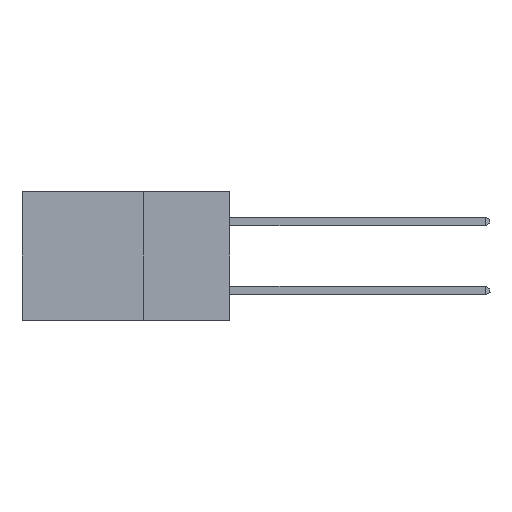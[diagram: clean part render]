
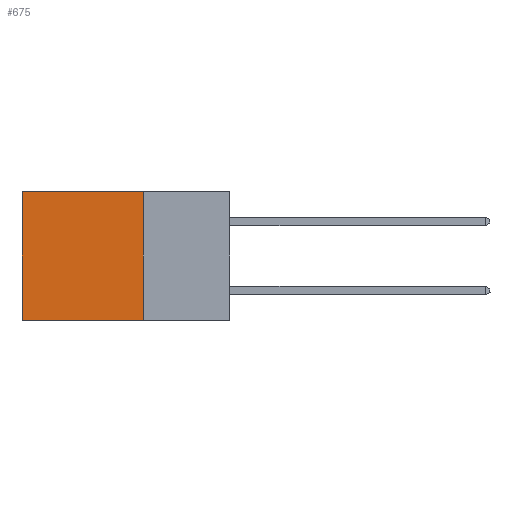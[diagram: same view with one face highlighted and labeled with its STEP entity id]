
A CAD part, left-side view. The second image highlights one B-rep face of the part: STEP entity #675.
In plain terms, the highlighted planar face has unit normal (-1, 0, 0).
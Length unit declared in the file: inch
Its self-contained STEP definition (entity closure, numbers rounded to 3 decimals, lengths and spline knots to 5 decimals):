
#675 = ADVANCED_FACE ( 'NONE', ( #4639 ), #16794, .F. ) ;
#2197 = DIRECTION ( 'NONE',  ( 0., 0., -1. ) ) ;
#4047 = LINE ( 'NONE', #15879, #23163 ) ;
#4639 = FACE_OUTER_BOUND ( 'NONE', #23449, .T. ) ;
#4798 = DIRECTION ( 'NONE',  ( 0., 0., -1. ) ) ;
#4952 = CARTESIAN_POINT ( 'NONE',  ( 0.298, 0.25, 0. ) ) ;
#5358 = CARTESIAN_POINT ( 'NONE',  ( 0.298, 0.25, -0.37 ) ) ;
#7124 = EDGE_CURVE ( 'NONE', #12856, #16286, #12184, .T. ) ;
#8109 = LINE ( 'NONE', #5358, #14785 ) ;
#8174 = CARTESIAN_POINT ( 'NONE',  ( 0.298, 0.25, -0.37 ) ) ;
#8877 = ORIENTED_EDGE ( 'NONE', *, *, #7124, .T. ) ;
#10805 = ORIENTED_EDGE ( 'NONE', *, *, #18701, .F. ) ;
#10984 = CARTESIAN_POINT ( 'NONE',  ( 0.298, 0.6, 0. ) ) ;
#11376 = DIRECTION ( 'NONE',  ( 1., 0., 0. ) ) ;
#11616 = VECTOR ( 'NONE', #12182, 39.37008 ) ;
#11776 = LINE ( 'NONE', #17432, #21935 ) ;
#12182 = DIRECTION ( 'NONE',  ( 0., 1., 0. ) ) ;
#12184 = LINE ( 'NONE', #17795, #11616 ) ;
#12258 = ORIENTED_EDGE ( 'NONE', *, *, #13973, .T. ) ;
#12856 = VERTEX_POINT ( 'NONE', #4952 ) ;
#12937 = DIRECTION ( 'NONE',  ( 0., 1., 0. ) ) ;
#13973 = EDGE_CURVE ( 'NONE', #16286, #21240, #4047, .T. ) ;
#14785 = VECTOR ( 'NONE', #12937, 39.37008 ) ;
#15267 = CARTESIAN_POINT ( 'NONE',  ( 0.298, 0.25, 0. ) ) ;
#15879 = CARTESIAN_POINT ( 'NONE',  ( 0.298, 0.6, 0. ) ) ;
#15997 = EDGE_CURVE ( 'NONE', #20125, #21240, #8109, .T. ) ;
#16286 = VERTEX_POINT ( 'NONE', #10984 ) ;
#16794 = PLANE ( 'NONE',  #23668 ) ;
#17432 = CARTESIAN_POINT ( 'NONE',  ( 0.298, 0.25, 0. ) ) ;
#17795 = CARTESIAN_POINT ( 'NONE',  ( 0.298, 0.25, 0. ) ) ;
#18701 = EDGE_CURVE ( 'NONE', #12856, #20125, #11776, .T. ) ;
#20125 = VERTEX_POINT ( 'NONE', #8174 ) ;
#21240 = VERTEX_POINT ( 'NONE', #21418 ) ;
#21261 = DIRECTION ( 'NONE',  ( 0., 0., -1. ) ) ;
#21418 = CARTESIAN_POINT ( 'NONE',  ( 0.298, 0.6, -0.37 ) ) ;
#21804 = ORIENTED_EDGE ( 'NONE', *, *, #15997, .F. ) ;
#21935 = VECTOR ( 'NONE', #21261, 39.37008 ) ;
#23163 = VECTOR ( 'NONE', #4798, 39.37008 ) ;
#23449 = EDGE_LOOP ( 'NONE', ( #12258, #21804, #10805, #8877 ) ) ;
#23668 = AXIS2_PLACEMENT_3D ( 'NONE', #15267, #11376, #2197 ) ;
